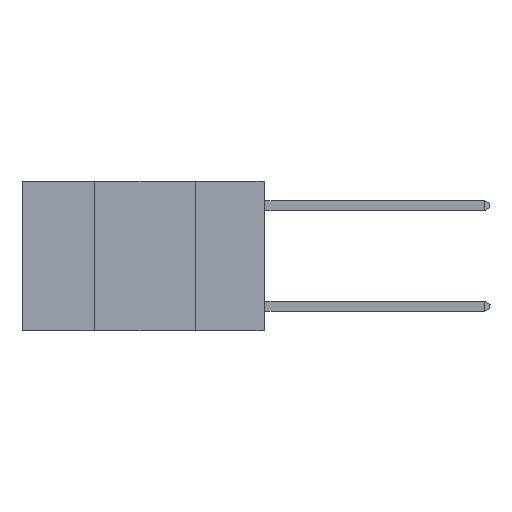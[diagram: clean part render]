
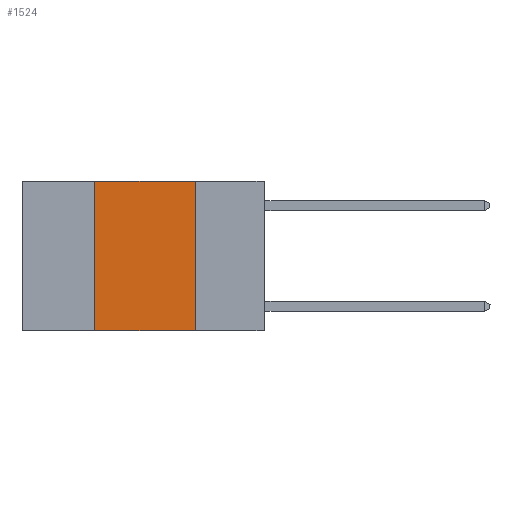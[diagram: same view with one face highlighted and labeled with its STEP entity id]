
A CAD part, left-side view. The second image highlights one B-rep face of the part: STEP entity #1524.
In plain terms, the highlighted planar face has unit normal (-1, 0, 0).
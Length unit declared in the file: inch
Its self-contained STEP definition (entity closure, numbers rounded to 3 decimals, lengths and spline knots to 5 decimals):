
#278 = EDGE_LOOP ( 'NONE', ( #6525, #1294, #6697, #3159 ) ) ;
#549 = DIRECTION ( 'NONE',  ( 1., 0., 0. ) ) ;
#673 = CARTESIAN_POINT ( 'NONE',  ( 0., 0.42, 0. ) ) ;
#1294 = ORIENTED_EDGE ( 'NONE', *, *, #17168, .F. ) ;
#1488 = CARTESIAN_POINT ( 'NONE',  ( 0., 0.17, 0. ) ) ;
#1524 = ADVANCED_FACE ( 'NONE', ( #7693 ), #11899, .F. ) ;
#2062 = DIRECTION ( 'NONE',  ( 0., 0., 1. ) ) ;
#2598 = VECTOR ( 'NONE', #3770, 39.37008 ) ;
#3159 = ORIENTED_EDGE ( 'NONE', *, *, #17592, .T. ) ;
#3420 = DIRECTION ( 'NONE',  ( 0., -1., 0. ) ) ;
#3518 = VECTOR ( 'NONE', #3420, 39.37008 ) ;
#3770 = DIRECTION ( 'NONE',  ( 0., -1., 0. ) ) ;
#5031 = LINE ( 'NONE', #673, #5710 ) ;
#5710 = VECTOR ( 'NONE', #2062, 39.37008 ) ;
#6525 = ORIENTED_EDGE ( 'NONE', *, *, #11633, .F. ) ;
#6697 = ORIENTED_EDGE ( 'NONE', *, *, #13339, .F. ) ;
#7492 = LINE ( 'NONE', #11704, #15518 ) ;
#7693 = FACE_OUTER_BOUND ( 'NONE', #278, .T. ) ;
#9082 = LINE ( 'NONE', #17717, #3518 ) ;
#9528 = CARTESIAN_POINT ( 'NONE',  ( 0., 0.6, 0. ) ) ;
#9902 = VERTEX_POINT ( 'NONE', #10927 ) ;
#10849 = LINE ( 'NONE', #9528, #2598 ) ;
#10927 = CARTESIAN_POINT ( 'NONE',  ( 0., 0.42, 0. ) ) ;
#11633 = EDGE_CURVE ( 'NONE', #12303, #12574, #7492, .T. ) ;
#11704 = CARTESIAN_POINT ( 'NONE',  ( 0., 0.17, 0. ) ) ;
#11899 = PLANE ( 'NONE',  #13222 ) ;
#12266 = CARTESIAN_POINT ( 'NONE',  ( 0., 0.17, -0.37 ) ) ;
#12303 = VERTEX_POINT ( 'NONE', #1488 ) ;
#12574 = VERTEX_POINT ( 'NONE', #12266 ) ;
#13222 = AXIS2_PLACEMENT_3D ( 'NONE', #14822, #549, #13397 ) ;
#13339 = EDGE_CURVE ( 'NONE', #14903, #9902, #5031, .T. ) ;
#13397 = DIRECTION ( 'NONE',  ( 0., 0., -1. ) ) ;
#14822 = CARTESIAN_POINT ( 'NONE',  ( 0., 0.6, 0. ) ) ;
#14903 = VERTEX_POINT ( 'NONE', #18377 ) ;
#15518 = VECTOR ( 'NONE', #16112, 39.37008 ) ;
#16112 = DIRECTION ( 'NONE',  ( 0., 0., -1. ) ) ;
#17168 = EDGE_CURVE ( 'NONE', #9902, #12303, #10849, .T. ) ;
#17592 = EDGE_CURVE ( 'NONE', #14903, #12574, #9082, .T. ) ;
#17717 = CARTESIAN_POINT ( 'NONE',  ( 0., 0.6, -0.37 ) ) ;
#18377 = CARTESIAN_POINT ( 'NONE',  ( 0., 0.42, -0.37 ) ) ;
